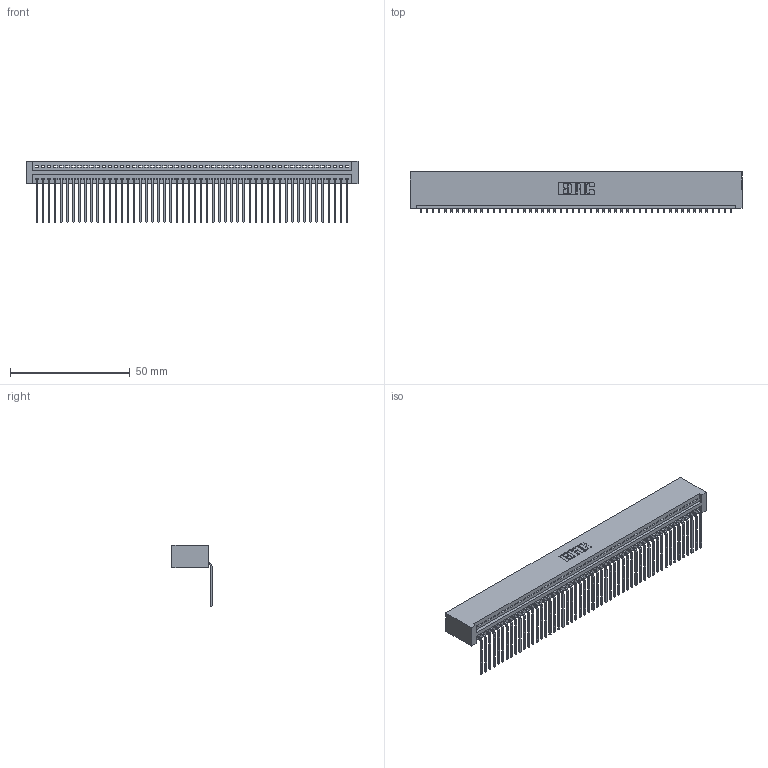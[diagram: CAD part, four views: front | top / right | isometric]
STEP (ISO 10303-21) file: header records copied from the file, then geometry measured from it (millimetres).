
FILE_DESCRIPTION (( 'STEP AP203' ), '1' );
FILE_NAME ('345-052-559-101.STEP', '2019-10-09T19:30:22', ( '' ), ( '' ), 'SwSTEP 2.0', 'SolidWorks 2016', '' );
FILE_SCHEMA (( 'CONFIG_CONTROL_DESIGN' ));
Length unit declared in the file: inch
Products named in the file (3): 345 Part_No Mounting Lugs; 345-052-559-101; 345-292-001_558 559 Tail - 1
Assembly tree (53 placements, depth 2):
  345-052-559-101
    345 Part_No Mounting Lugs
    345-292-001_558 559 Tail - 1  x52
Bounding box: 138.68 x 16.75 x 25.53 mm (x, y, z)
Volume: 14011.9 mm3; surface area: 19964.6 mm2
Topology: 53 solids, 53 shells, 3238 faces, 9781 edges, 6450 vertices
Faces by surface type: plane 2260, cylinder 978
Entity records: 37597 total; most frequent: CARTESIAN_POINT 6520, ORIENTED_EDGE 6506, DIRECTION 5673, EDGE_CURVE 3253, LINE 2921, VECTOR 2921, VERTEX_POINT 2166, AXIS2_PLACEMENT_3D 1376
